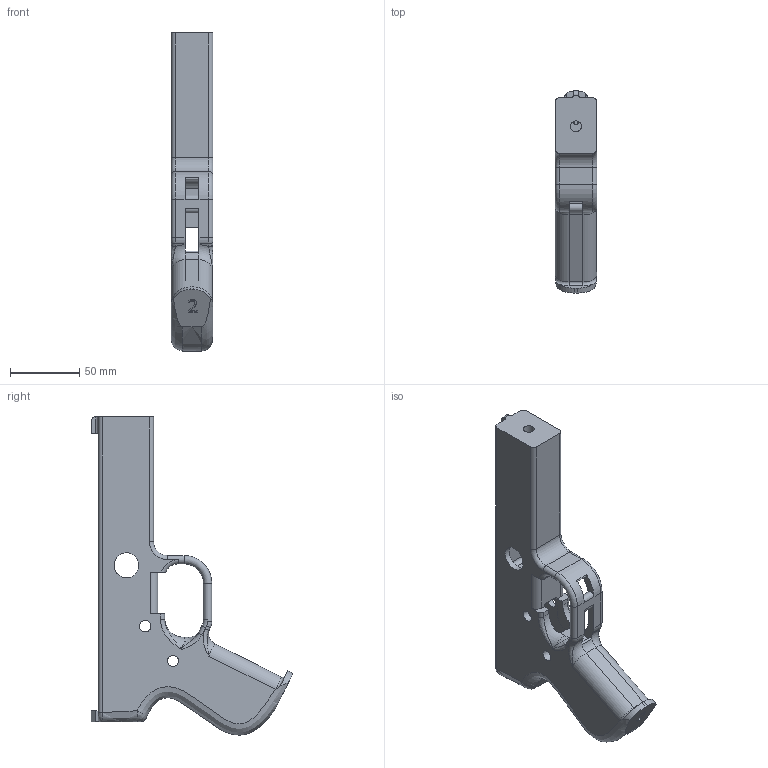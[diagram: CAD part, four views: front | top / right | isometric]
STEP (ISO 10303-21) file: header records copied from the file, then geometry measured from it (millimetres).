
FILE_DESCRIPTION((''),'2;1');
FILE_NAME('PM422Frame2.stp','2015-09-29T15:53:02',('JamesRPatrick'),(''),'Autodesk Inventor 2012','Autodesk Inventor 2012','');
FILE_SCHEMA(('AUTOMOTIVE_DESIGN { 1 0 10303 214 1 1 1 1 }'));
Length unit declared in the file: millimetre
Products named in the file (1): PM422Frame2
Bounding box: 30 x 145.5 x 229.5 mm (x, y, z)
Volume: 228846.8 mm3; surface area: 71565.7 mm2
Topology: 1 solids, 1 shells, 577 faces, 1593 edges, 1032 vertices
Faces by surface type: plane 269, bspline 182, cylinder 92, torus 30, sphere 4
Full cylindrical faces by diameter (mm): 3 x1, 8 x1, 8.1 x4, 12 x3, 18 x1
Entity records: 21304 total; most frequent: CARTESIAN_POINT 7457, ORIENTED_EDGE 3148, DIRECTION 2206, EDGE_CURVE 1574, VERTEX_POINT 1027, VECTOR 916, LINE 916, AXIS2_PLACEMENT_3D 645
